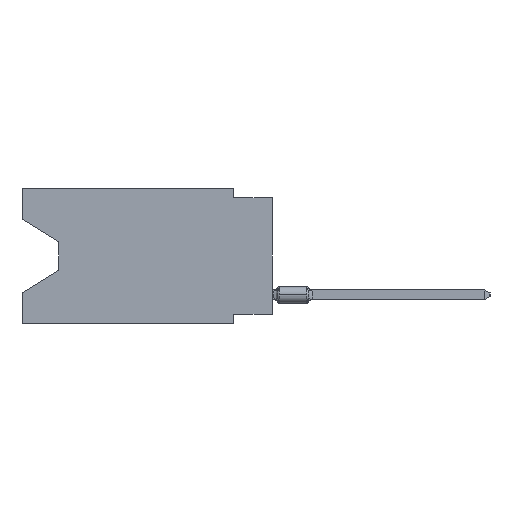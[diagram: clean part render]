
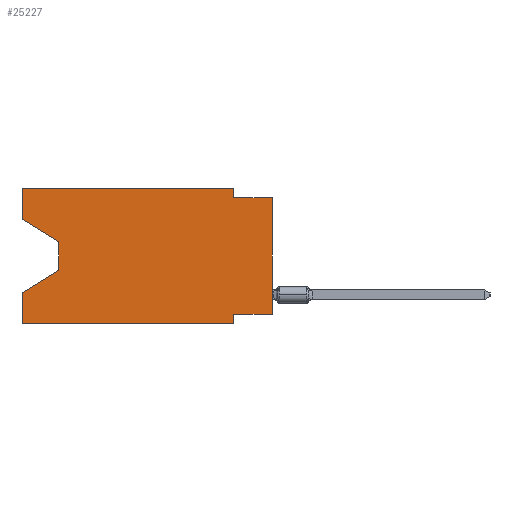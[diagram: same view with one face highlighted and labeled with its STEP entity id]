
A CAD part, left-side view. The second image highlights one B-rep face of the part: STEP entity #25227.
In plain terms, the highlighted planar face has unit normal (-1, 0, 0).
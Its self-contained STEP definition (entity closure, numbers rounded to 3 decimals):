
#331 = CARTESIAN_POINT ( 'NONE',  ( 0., 13.97, -3.505 ) ) ;
#661 = VECTOR ( 'NONE', #22259, 1000. ) ;
#1005 = PLANE ( 'NONE',  #24007 ) ;
#1058 = CARTESIAN_POINT ( 'NONE',  ( 0., 2.54, -8.255 ) ) ;
#1250 = EDGE_CURVE ( 'NONE', #14175, #9868, #10071, .T. ) ;
#2233 = VERTEX_POINT ( 'NONE', #23517 ) ;
#2267 = DIRECTION ( 'NONE',  ( 0., 0., 1. ) ) ;
#2275 = ORIENTED_EDGE ( 'NONE', *, *, #22323, .F. ) ;
#2346 = ORIENTED_EDGE ( 'NONE', *, *, #9696, .F. ) ;
#2617 = VERTEX_POINT ( 'NONE', #26842 ) ;
#2692 = LINE ( 'NONE', #8927, #17836 ) ;
#2876 = VECTOR ( 'NONE', #12783, 1000. ) ;
#3594 = LINE ( 'NONE', #22324, #3682 ) ;
#3614 = LINE ( 'NONE', #9311, #11309 ) ;
#3682 = VECTOR ( 'NONE', #24543, 1000. ) ;
#3700 = VECTOR ( 'NONE', #6319, 1000. ) ;
#4094 = CARTESIAN_POINT ( 'NONE',  ( 0., 16.383, -8.89 ) ) ;
#5122 = EDGE_CURVE ( 'NONE', #20297, #26256, #11958, .T. ) ;
#5251 = VERTEX_POINT ( 'NONE', #18530 ) ;
#5336 = EDGE_CURVE ( 'NONE', #2233, #14175, #2692, .T. ) ;
#5709 = CARTESIAN_POINT ( 'NONE',  ( 0., 16.383, -2.038 ) ) ;
#6006 = VECTOR ( 'NONE', #12892, 1000. ) ;
#6319 = DIRECTION ( 'NONE',  ( 0., 0., 1. ) ) ;
#6833 = LINE ( 'NONE', #12933, #26657 ) ;
#7395 = CARTESIAN_POINT ( 'NONE',  ( 0., 16.383, 0. ) ) ;
#7704 = ORIENTED_EDGE ( 'NONE', *, *, #19445, .F. ) ;
#7705 = DIRECTION ( 'NONE',  ( 0., 0., 1. ) ) ;
#8305 = VERTEX_POINT ( 'NONE', #9702 ) ;
#8311 = LINE ( 'NONE', #10259, #12586 ) ;
#8427 = LINE ( 'NONE', #16903, #15959 ) ;
#8663 = DIRECTION ( 'NONE',  ( 0., 1., 0. ) ) ;
#8927 = CARTESIAN_POINT ( 'NONE',  ( 0., 0., -8.255 ) ) ;
#9194 = DIRECTION ( 'NONE',  ( 1., 0., 0. ) ) ;
#9311 = CARTESIAN_POINT ( 'NONE',  ( 0., 13.97, -3.505 ) ) ;
#9696 = EDGE_CURVE ( 'NONE', #2617, #5251, #25656, .T. ) ;
#9702 = CARTESIAN_POINT ( 'NONE',  ( 0., 0., -0.635 ) ) ;
#9868 = VERTEX_POINT ( 'NONE', #20105 ) ;
#10071 = LINE ( 'NONE', #17092, #2876 ) ;
#10098 = LINE ( 'NONE', #26994, #3700 ) ;
#10259 = CARTESIAN_POINT ( 'NONE',  ( 0., 0., -0.635 ) ) ;
#10260 = ORIENTED_EDGE ( 'NONE', *, *, #18375, .T. ) ;
#11281 = FACE_OUTER_BOUND ( 'NONE', #18589, .T. ) ;
#11309 = VECTOR ( 'NONE', #26374, 1000. ) ;
#11868 = LINE ( 'NONE', #22527, #661 ) ;
#11872 = LINE ( 'NONE', #22264, #15003 ) ;
#11958 = LINE ( 'NONE', #5709, #18704 ) ;
#12392 = ORIENTED_EDGE ( 'NONE', *, *, #20437, .T. ) ;
#12450 = ORIENTED_EDGE ( 'NONE', *, *, #17792, .T. ) ;
#12586 = VECTOR ( 'NONE', #18584, 1000. ) ;
#12783 = DIRECTION ( 'NONE',  ( 0., 0., -1. ) ) ;
#12892 = DIRECTION ( 'NONE',  ( 0., -1., 0. ) ) ;
#12933 = CARTESIAN_POINT ( 'NONE',  ( 0., 16.383, 0. ) ) ;
#13203 = CARTESIAN_POINT ( 'NONE',  ( 0., 16.383, -2.038 ) ) ;
#14175 = VERTEX_POINT ( 'NONE', #1058 ) ;
#14197 = EDGE_CURVE ( 'NONE', #17148, #20177, #11872, .T. ) ;
#14369 = ORIENTED_EDGE ( 'NONE', *, *, #1250, .F. ) ;
#14426 = CARTESIAN_POINT ( 'NONE',  ( 0., 13.97, -5.385 ) ) ;
#14832 = DIRECTION ( 'NONE',  ( 0., 0., -1. ) ) ;
#15003 = VECTOR ( 'NONE', #7705, 1000. ) ;
#15867 = DIRECTION ( 'NONE',  ( 0., 0., -1. ) ) ;
#15959 = VECTOR ( 'NONE', #14832, 1000. ) ;
#16076 = EDGE_CURVE ( 'NONE', #16787, #20177, #11868, .T. ) ;
#16787 = VERTEX_POINT ( 'NONE', #14426 ) ;
#16903 = CARTESIAN_POINT ( 'NONE',  ( 0., 2.54, 0. ) ) ;
#17092 = CARTESIAN_POINT ( 'NONE',  ( 0., 2.54, -8.89 ) ) ;
#17148 = VERTEX_POINT ( 'NONE', #4094 ) ;
#17792 = EDGE_CURVE ( 'NONE', #17148, #9868, #3594, .T. ) ;
#17836 = VECTOR ( 'NONE', #8663, 1000. ) ;
#18375 = EDGE_CURVE ( 'NONE', #2233, #8305, #10098, .T. ) ;
#18530 = CARTESIAN_POINT ( 'NONE',  ( 0., 2.54, 0. ) ) ;
#18584 = DIRECTION ( 'NONE',  ( 0., -1., 0. ) ) ;
#18589 = EDGE_LOOP ( 'NONE', ( #23966, #12392, #21145, #22646, #12450, #14369, #22263, #10260, #7704, #2275, #2346, #18825 ) ) ;
#18621 = CARTESIAN_POINT ( 'NONE',  ( 0., 16.383, -6.852 ) ) ;
#18704 = VECTOR ( 'NONE', #24306, 1000. ) ;
#18825 = ORIENTED_EDGE ( 'NONE', *, *, #25017, .F. ) ;
#19445 = EDGE_CURVE ( 'NONE', #24159, #8305, #8311, .T. ) ;
#20105 = CARTESIAN_POINT ( 'NONE',  ( 0., 2.54, -8.89 ) ) ;
#20177 = VERTEX_POINT ( 'NONE', #18621 ) ;
#20297 = VERTEX_POINT ( 'NONE', #13203 ) ;
#20437 = EDGE_CURVE ( 'NONE', #26256, #16787, #3614, .T. ) ;
#21145 = ORIENTED_EDGE ( 'NONE', *, *, #16076, .T. ) ;
#21881 = CARTESIAN_POINT ( 'NONE',  ( 0., 2.54, -0.635 ) ) ;
#22259 = DIRECTION ( 'NONE',  ( 0., 0.855, -0.519 ) ) ;
#22263 = ORIENTED_EDGE ( 'NONE', *, *, #5336, .F. ) ;
#22264 = CARTESIAN_POINT ( 'NONE',  ( 0., 16.383, 0. ) ) ;
#22323 = EDGE_CURVE ( 'NONE', #5251, #24159, #8427, .T. ) ;
#22324 = CARTESIAN_POINT ( 'NONE',  ( 0., 16.383, -8.89 ) ) ;
#22527 = CARTESIAN_POINT ( 'NONE',  ( 0., 13.97, -5.385 ) ) ;
#22646 = ORIENTED_EDGE ( 'NONE', *, *, #14197, .F. ) ;
#23517 = CARTESIAN_POINT ( 'NONE',  ( 0., 0., -8.255 ) ) ;
#23843 = CARTESIAN_POINT ( 'NONE',  ( 0., 16.383, 0. ) ) ;
#23966 = ORIENTED_EDGE ( 'NONE', *, *, #5122, .T. ) ;
#24007 = AXIS2_PLACEMENT_3D ( 'NONE', #7395, #9194, #15867 ) ;
#24159 = VERTEX_POINT ( 'NONE', #21881 ) ;
#24306 = DIRECTION ( 'NONE',  ( 0., -0.855, -0.519 ) ) ;
#24543 = DIRECTION ( 'NONE',  ( 0., -1., 0. ) ) ;
#25017 = EDGE_CURVE ( 'NONE', #20297, #2617, #6833, .T. ) ;
#25227 = ADVANCED_FACE ( 'NONE', ( #11281 ), #1005, .F. ) ;
#25656 = LINE ( 'NONE', #23843, #6006 ) ;
#26256 = VERTEX_POINT ( 'NONE', #331 ) ;
#26374 = DIRECTION ( 'NONE',  ( 0., 0., -1. ) ) ;
#26657 = VECTOR ( 'NONE', #2267, 1000. ) ;
#26842 = CARTESIAN_POINT ( 'NONE',  ( 0., 16.383, 0. ) ) ;
#26994 = CARTESIAN_POINT ( 'NONE',  ( 0., 0., 0. ) ) ;
